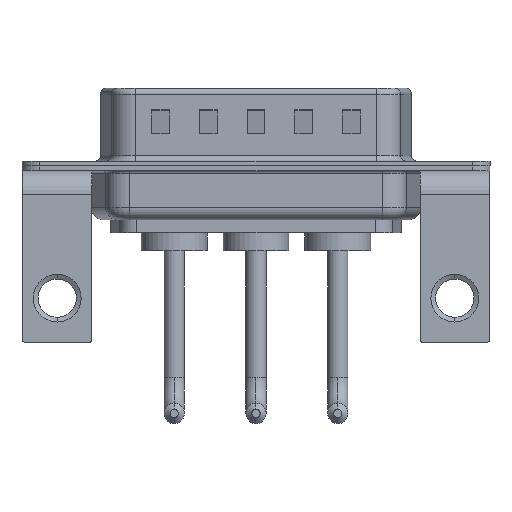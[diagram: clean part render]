
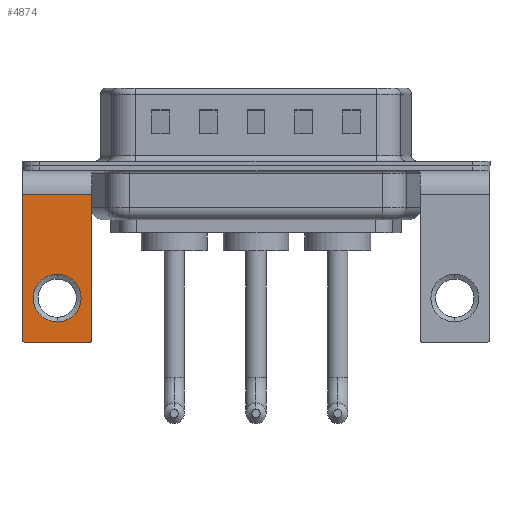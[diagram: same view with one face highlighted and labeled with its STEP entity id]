
A CAD part, front view. The second image highlights one B-rep face of the part: STEP entity #4874.
In plain terms, the highlighted planar face has unit normal (0, -1, 0).
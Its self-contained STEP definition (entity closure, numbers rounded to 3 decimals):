
#491 = CARTESIAN_POINT ( 'NONE',  ( 0., -6.25, -13.07 ) ) ;
#548 = DIRECTION ( 'NONE',  ( 0., 1., 0. ) ) ;
#635 = PLANE ( 'NONE',  #16452 ) ;
#737 = CARTESIAN_POINT ( 'NONE',  ( 2.65, -6.25, -14.8 ) ) ;
#817 = DIRECTION ( 'NONE',  ( 0., -1., 0. ) ) ;
#871 = LINE ( 'NONE', #4621, #14732 ) ;
#944 = EDGE_CURVE ( 'NONE', #10866, #15384, #1009, .T. ) ;
#1009 = CIRCLE ( 'NONE', #16592, 2. ) ;
#1283 = EDGE_LOOP ( 'NONE', ( #2781, #4272, #15500, #15118, #14217, #4111 ) ) ;
#1307 = CIRCLE ( 'NONE', #15272, 2. ) ;
#1896 = CARTESIAN_POINT ( 'NONE',  ( 2.9, -6.25, -14.8 ) ) ;
#2085 = DIRECTION ( 'NONE',  ( 0., 0., 1. ) ) ;
#2185 = DIRECTION ( 'NONE',  ( 0., 1., 0. ) ) ;
#2781 = ORIENTED_EDGE ( 'NONE', *, *, #11773, .T. ) ;
#3007 = CARTESIAN_POINT ( 'NONE',  ( 0., -6.25, -11.07 ) ) ;
#3038 = VERTEX_POINT ( 'NONE', #737 ) ;
#3223 = DIRECTION ( 'NONE',  ( -1., 0., 0. ) ) ;
#3268 = DIRECTION ( 'NONE',  ( 0., 0., 1. ) ) ;
#3392 = CARTESIAN_POINT ( 'NONE',  ( 2.65, -6.25, -14.55 ) ) ;
#3420 = CARTESIAN_POINT ( 'NONE',  ( 2.9, -6.25, -14.55 ) ) ;
#4111 = ORIENTED_EDGE ( 'NONE', *, *, #16644, .T. ) ;
#4138 = CARTESIAN_POINT ( 'NONE',  ( 0., -6.25, -9.07 ) ) ;
#4272 = ORIENTED_EDGE ( 'NONE', *, *, #4301, .T. ) ;
#4294 = CARTESIAN_POINT ( 'NONE',  ( 2.9, -6.25, -2.4 ) ) ;
#4301 = EDGE_CURVE ( 'NONE', #7629, #6242, #15871, .T. ) ;
#4364 = EDGE_CURVE ( 'NONE', #3038, #5996, #10473, .T. ) ;
#4621 = CARTESIAN_POINT ( 'NONE',  ( 2.9, -6.25, -2.4 ) ) ;
#4713 = CARTESIAN_POINT ( 'NONE',  ( -2.9, -6.25, -2.4 ) ) ;
#4874 = ADVANCED_FACE ( 'NONE', ( #5618, #14761 ), #635, .F. ) ;
#5030 = EDGE_LOOP ( 'NONE', ( #10413, #13495 ) ) ;
#5618 = FACE_BOUND ( 'NONE', #5030, .T. ) ;
#5725 = DIRECTION ( 'NONE',  ( 0., 0., 1. ) ) ;
#5879 = AXIS2_PLACEMENT_3D ( 'NONE', #3392, #817, #8250 ) ;
#5996 = VERTEX_POINT ( 'NONE', #3420 ) ;
#6242 = VERTEX_POINT ( 'NONE', #7748 ) ;
#6890 = VECTOR ( 'NONE', #3223, 1000. ) ;
#7062 = VERTEX_POINT ( 'NONE', #4713 ) ;
#7123 = DIRECTION ( 'NONE',  ( 0., 0., 1. ) ) ;
#7160 = DIRECTION ( 'NONE',  ( 0., 1., 0. ) ) ;
#7629 = VERTEX_POINT ( 'NONE', #11602 ) ;
#7748 = CARTESIAN_POINT ( 'NONE',  ( -2.65, -6.25, -14.8 ) ) ;
#8116 = CARTESIAN_POINT ( 'NONE',  ( -2.9, -6.25, -2.4 ) ) ;
#8186 = VERTEX_POINT ( 'NONE', #14619 ) ;
#8250 = DIRECTION ( 'NONE',  ( 0., 0., 1. ) ) ;
#8311 = EDGE_CURVE ( 'NONE', #3038, #6242, #9601, .T. ) ;
#8790 = EDGE_CURVE ( 'NONE', #8186, #5996, #871, .T. ) ;
#9277 = EDGE_CURVE ( 'NONE', #15384, #10866, #1307, .T. ) ;
#9379 = LINE ( 'NONE', #8116, #11026 ) ;
#9601 = LINE ( 'NONE', #1896, #6890 ) ;
#9831 = DIRECTION ( 'NONE',  ( 0., 0., -1. ) ) ;
#10029 = VECTOR ( 'NONE', #12674, 1000. ) ;
#10058 = LINE ( 'NONE', #15224, #10029 ) ;
#10413 = ORIENTED_EDGE ( 'NONE', *, *, #944, .T. ) ;
#10473 = CIRCLE ( 'NONE', #5879, 0.25 ) ;
#10866 = VERTEX_POINT ( 'NONE', #491 ) ;
#11026 = VECTOR ( 'NONE', #13285, 1000. ) ;
#11169 = CARTESIAN_POINT ( 'NONE',  ( 0., -6.25, -11.07 ) ) ;
#11602 = CARTESIAN_POINT ( 'NONE',  ( -2.9, -6.25, -14.55 ) ) ;
#11773 = EDGE_CURVE ( 'NONE', #7062, #7629, #9379, .T. ) ;
#12674 = DIRECTION ( 'NONE',  ( -1., 0., 0. ) ) ;
#13285 = DIRECTION ( 'NONE',  ( 0., 0., -1. ) ) ;
#13445 = AXIS2_PLACEMENT_3D ( 'NONE', #14869, #13601, #5725 ) ;
#13495 = ORIENTED_EDGE ( 'NONE', *, *, #9277, .T. ) ;
#13601 = DIRECTION ( 'NONE',  ( 0., -1., 0. ) ) ;
#14217 = ORIENTED_EDGE ( 'NONE', *, *, #8790, .F. ) ;
#14619 = CARTESIAN_POINT ( 'NONE',  ( 2.9, -6.25, -2.4 ) ) ;
#14732 = VECTOR ( 'NONE', #9831, 1000. ) ;
#14761 = FACE_OUTER_BOUND ( 'NONE', #1283, .T. ) ;
#14869 = CARTESIAN_POINT ( 'NONE',  ( -2.65, -6.25, -14.55 ) ) ;
#15118 = ORIENTED_EDGE ( 'NONE', *, *, #4364, .T. ) ;
#15224 = CARTESIAN_POINT ( 'NONE',  ( 2.9, -6.25, -2.4 ) ) ;
#15272 = AXIS2_PLACEMENT_3D ( 'NONE', #11169, #2185, #3268 ) ;
#15384 = VERTEX_POINT ( 'NONE', #4138 ) ;
#15500 = ORIENTED_EDGE ( 'NONE', *, *, #8311, .F. ) ;
#15871 = CIRCLE ( 'NONE', #13445, 0.25 ) ;
#16452 = AXIS2_PLACEMENT_3D ( 'NONE', #4294, #548, #7123 ) ;
#16592 = AXIS2_PLACEMENT_3D ( 'NONE', #3007, #7160, #2085 ) ;
#16644 = EDGE_CURVE ( 'NONE', #8186, #7062, #10058, .T. ) ;
